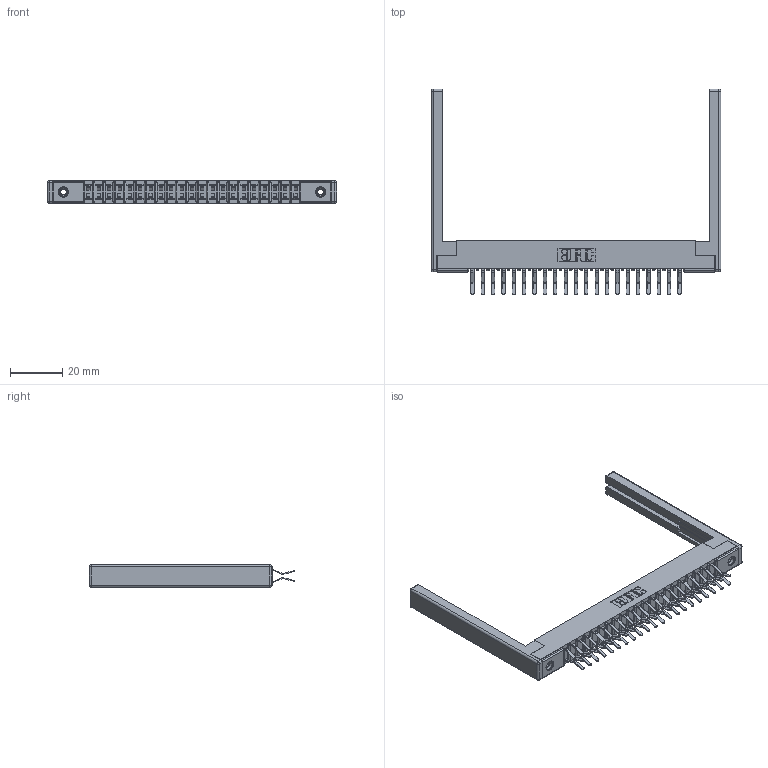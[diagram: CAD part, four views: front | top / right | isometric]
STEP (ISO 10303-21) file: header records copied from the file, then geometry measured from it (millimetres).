
FILE_DESCRIPTION (( 'STEP AP203' ), '1' );
FILE_NAME ('357-042-460-268.STEP', '2020-10-03T23:20:19', ( '' ), ( '' ), 'SwSTEP 2.0', 'SolidWorks 2020', '' );
FILE_SCHEMA (( 'CONFIG_CONTROL_DESIGN' ));
Length unit declared in the file: inch
Products named in the file (5): 345-250-001_345-250-001-102; 357-042-460-268; 307-290-001_560; 307-220-068; 307 Part_.156 Dia Mounting Holes
Assembly tree (47 placements, depth 2):
  357-042-460-268
    307 Part_.156 Dia Mounting Holes
    307-290-001_560  x42
    307-220-068  x2
    345-250-001_345-250-001-102  x2
Bounding box: 110.64 x 78.69 x 8.71 mm (x, y, z)
Volume: 11851.1 mm3; surface area: 17185 mm2
Topology: 47 solids, 47 shells, 2394 faces, 6677 edges, 4314 vertices
Faces by surface type: plane 1544, cylinder 782, sphere 52, cone 12, torus 4
Entity records: 24127 total; most frequent: CARTESIAN_POINT 3930, ORIENTED_EDGE 3884, DIRECTION 3874, EDGE_CURVE 1942, VECTOR 1478, LINE 1478, VERTEX_POINT 1254, AXIS2_PLACEMENT_3D 1198
